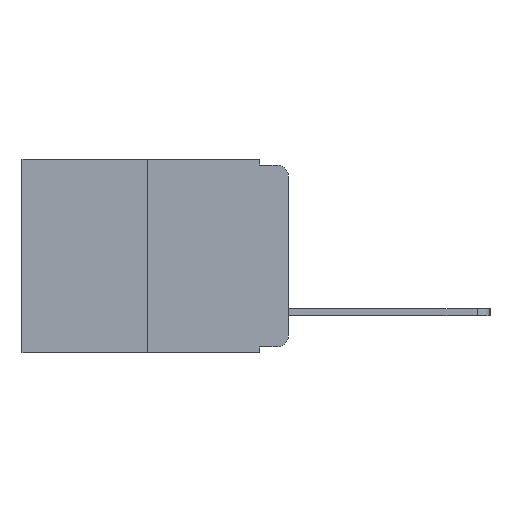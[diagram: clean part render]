
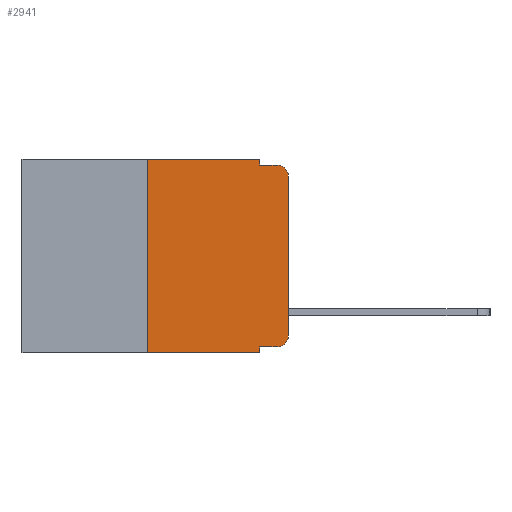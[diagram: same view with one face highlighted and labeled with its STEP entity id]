
A CAD part, left-side view. The second image highlights one B-rep face of the part: STEP entity #2941.
In plain terms, the highlighted planar face has unit normal (-1, 0, 0).
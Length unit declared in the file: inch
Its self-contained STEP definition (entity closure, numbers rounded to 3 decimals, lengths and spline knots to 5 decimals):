
#155 = DIRECTION ( 'NONE',  ( 0., 0., 1. ) ) ;
#267 = VECTOR ( 'NONE', #4971, 39.37008 ) ;
#610 = VERTEX_POINT ( 'NONE', #7967 ) ;
#682 = CARTESIAN_POINT ( 'NONE',  ( 0., 0.051, -0.333 ) ) ;
#752 = ORIENTED_EDGE ( 'NONE', *, *, #14256, .F. ) ;
#1056 = ORIENTED_EDGE ( 'NONE', *, *, #16058, .F. ) ;
#1149 = VECTOR ( 'NONE', #155, 39.37008 ) ;
#1209 = EDGE_CURVE ( 'NONE', #20503, #5442, #17486, .T. ) ;
#1545 = CARTESIAN_POINT ( 'NONE',  ( 0., 0.02, -0.03 ) ) ;
#1704 = DIRECTION ( 'NONE',  ( 0., 0., -1. ) ) ;
#2151 = CARTESIAN_POINT ( 'NONE',  ( 0., 0.051, 0. ) ) ;
#2191 = EDGE_CURVE ( 'NONE', #610, #20503, #5340, .T. ) ;
#2284 = ORIENTED_EDGE ( 'NONE', *, *, #12255, .F. ) ;
#2300 = LINE ( 'NONE', #3065, #19675 ) ;
#2345 = CARTESIAN_POINT ( 'NONE',  ( 0., 0.051, -0.333 ) ) ;
#2397 = LINE ( 'NONE', #682, #10626 ) ;
#2480 = CARTESIAN_POINT ( 'NONE',  ( 0., 0.02, -0.313 ) ) ;
#2859 = ORIENTED_EDGE ( 'NONE', *, *, #5256, .F. ) ;
#2941 = ADVANCED_FACE ( 'NONE', ( #15878 ), #16733, .F. ) ;
#3065 = CARTESIAN_POINT ( 'NONE',  ( 0., 0.051, -0.01 ) ) ;
#3191 = CARTESIAN_POINT ( 'NONE',  ( 0., 0.473, 0. ) ) ;
#3234 = VECTOR ( 'NONE', #13602, 39.37008 ) ;
#3427 = DIRECTION ( 'NONE',  ( 0., 0., -1. ) ) ;
#4283 = DIRECTION ( 'NONE',  ( 0., 0., -1. ) ) ;
#4315 = LINE ( 'NONE', #10020, #7589 ) ;
#4565 = EDGE_CURVE ( 'NONE', #6781, #610, #2397, .T. ) ;
#4698 = VERTEX_POINT ( 'NONE', #20688 ) ;
#4796 = AXIS2_PLACEMENT_3D ( 'NONE', #10374, #8744, #15115 ) ;
#4971 = DIRECTION ( 'NONE',  ( 0., -1., 0. ) ) ;
#5123 = LINE ( 'NONE', #3191, #267 ) ;
#5256 = EDGE_CURVE ( 'NONE', #4698, #11406, #6365, .T. ) ;
#5340 = CIRCLE ( 'NONE', #12140, 0.02 ) ;
#5442 = VERTEX_POINT ( 'NONE', #5886 ) ;
#5578 = DIRECTION ( 'NONE',  ( 0., 0., 1. ) ) ;
#5755 = CARTESIAN_POINT ( 'NONE',  ( 0., 0.02, -0.01 ) ) ;
#5779 = ORIENTED_EDGE ( 'NONE', *, *, #13845, .F. ) ;
#5886 = CARTESIAN_POINT ( 'NONE',  ( 0., 0., -0.03 ) ) ;
#6365 = LINE ( 'NONE', #20070, #1149 ) ;
#6420 = CARTESIAN_POINT ( 'NONE',  ( 0., 0.25, 0. ) ) ;
#6781 = VERTEX_POINT ( 'NONE', #2345 ) ;
#7406 = CARTESIAN_POINT ( 'NONE',  ( 0., 0.473, -0.343 ) ) ;
#7423 = VERTEX_POINT ( 'NONE', #10052 ) ;
#7589 = VECTOR ( 'NONE', #1704, 39.37008 ) ;
#7609 = LINE ( 'NONE', #2151, #3234 ) ;
#7939 = CARTESIAN_POINT ( 'NONE',  ( 0., 0., 0. ) ) ;
#7965 = EDGE_LOOP ( 'NONE', ( #15583, #16111, #1056, #5779, #2284, #2859, #12523, #752, #18427, #10786 ) ) ;
#7967 = CARTESIAN_POINT ( 'NONE',  ( 0., 0.02, -0.333 ) ) ;
#8075 = CARTESIAN_POINT ( 'NONE',  ( 0., 0.051, -0.01 ) ) ;
#8512 = VERTEX_POINT ( 'NONE', #5755 ) ;
#8744 = DIRECTION ( 'NONE',  ( 1., 0., 0. ) ) ;
#8912 = VERTEX_POINT ( 'NONE', #8075 ) ;
#10020 = CARTESIAN_POINT ( 'NONE',  ( 0., 0.051, 0. ) ) ;
#10052 = CARTESIAN_POINT ( 'NONE',  ( 0., 0.051, -0.343 ) ) ;
#10313 = VERTEX_POINT ( 'NONE', #10834 ) ;
#10374 = CARTESIAN_POINT ( 'NONE',  ( 0., 0.473, 0. ) ) ;
#10518 = VECTOR ( 'NONE', #15422, 39.37008 ) ;
#10626 = VECTOR ( 'NONE', #12396, 39.37008 ) ;
#10786 = ORIENTED_EDGE ( 'NONE', *, *, #2191, .T. ) ;
#10834 = CARTESIAN_POINT ( 'NONE',  ( 0., 0.051, 0. ) ) ;
#10891 = AXIS2_PLACEMENT_3D ( 'NONE', #1545, #13091, #3427 ) ;
#11406 = VERTEX_POINT ( 'NONE', #6420 ) ;
#12140 = AXIS2_PLACEMENT_3D ( 'NONE', #2480, #13885, #4283 ) ;
#12255 = EDGE_CURVE ( 'NONE', #11406, #10313, #5123, .T. ) ;
#12396 = DIRECTION ( 'NONE',  ( 0., -1., 0. ) ) ;
#12523 = ORIENTED_EDGE ( 'NONE', *, *, #15826, .T. ) ;
#13091 = DIRECTION ( 'NONE',  ( -1., 0., 0. ) ) ;
#13602 = DIRECTION ( 'NONE',  ( 0., 0., -1. ) ) ;
#13845 = EDGE_CURVE ( 'NONE', #10313, #8912, #7609, .T. ) ;
#13885 = DIRECTION ( 'NONE',  ( -1., 0., 0. ) ) ;
#14256 = EDGE_CURVE ( 'NONE', #6781, #7423, #4315, .T. ) ;
#14434 = CARTESIAN_POINT ( 'NONE',  ( 0., 0., -0.313 ) ) ;
#15115 = DIRECTION ( 'NONE',  ( 0., 0., -1. ) ) ;
#15326 = LINE ( 'NONE', #7406, #10518 ) ;
#15422 = DIRECTION ( 'NONE',  ( 0., -1., 0. ) ) ;
#15583 = ORIENTED_EDGE ( 'NONE', *, *, #1209, .T. ) ;
#15826 = EDGE_CURVE ( 'NONE', #4698, #7423, #15326, .T. ) ;
#15878 = FACE_OUTER_BOUND ( 'NONE', #7965, .T. ) ;
#16058 = EDGE_CURVE ( 'NONE', #8912, #8512, #2300, .T. ) ;
#16111 = ORIENTED_EDGE ( 'NONE', *, *, #18254, .T. ) ;
#16466 = VECTOR ( 'NONE', #5578, 39.37008 ) ;
#16733 = PLANE ( 'NONE',  #4796 ) ;
#17486 = LINE ( 'NONE', #7939, #16466 ) ;
#18254 = EDGE_CURVE ( 'NONE', #5442, #8512, #20805, .T. ) ;
#18427 = ORIENTED_EDGE ( 'NONE', *, *, #4565, .T. ) ;
#19675 = VECTOR ( 'NONE', #20849, 39.37008 ) ;
#20070 = CARTESIAN_POINT ( 'NONE',  ( 0., 0.25, 0. ) ) ;
#20503 = VERTEX_POINT ( 'NONE', #14434 ) ;
#20688 = CARTESIAN_POINT ( 'NONE',  ( 0., 0.25, -0.343 ) ) ;
#20805 = CIRCLE ( 'NONE', #10891, 0.02 ) ;
#20849 = DIRECTION ( 'NONE',  ( 0., -1., 0. ) ) ;
